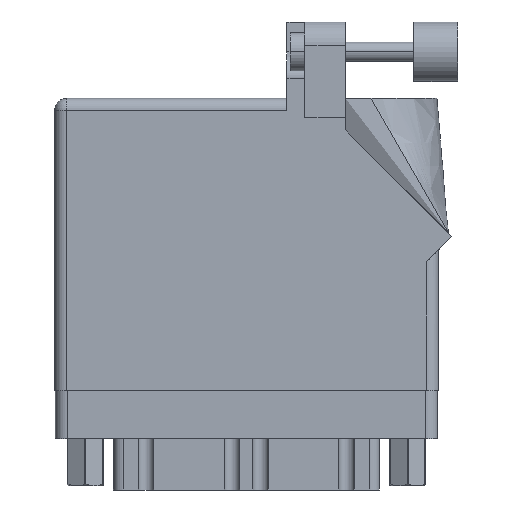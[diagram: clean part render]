
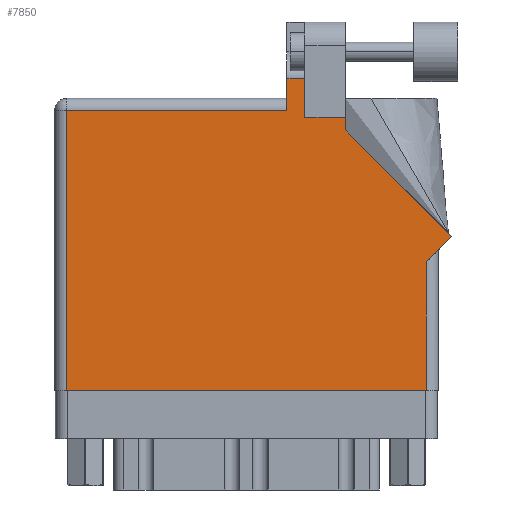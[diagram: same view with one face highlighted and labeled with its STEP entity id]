
A CAD part, front view. The second image highlights one B-rep face of the part: STEP entity #7850.
In plain terms, the highlighted face is planar.
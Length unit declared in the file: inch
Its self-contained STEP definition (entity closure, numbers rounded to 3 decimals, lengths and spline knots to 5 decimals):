
#1096 = CARTESIAN_POINT ( 'NONE',  ( 2.08071, 0.80771, 0. ) ) ;
#1359 = CARTESIAN_POINT ( 'NONE',  ( 1.64177, 1.6315, 0. ) ) ;
#1380 = DIRECTION ( 'NONE',  ( -0.707, 0.707, 0. ) ) ;
#2494 = ORIENTED_EDGE ( 'NONE', *, *, #47624, .T. ) ;
#3216 = ORIENTED_EDGE ( 'NONE', *, *, #21384, .T. ) ;
#3385 = CARTESIAN_POINT ( 'NONE',  ( 1.948, 0.675, 0. ) ) ;
#4133 = EDGE_CURVE ( 'NONE', #13836, #4342, #5826, .T. ) ;
#4342 = VERTEX_POINT ( 'NONE', #3385 ) ;
#4451 = LINE ( 'NONE', #30096, #24862 ) ;
#4482 = DIRECTION ( 'NONE',  ( -1., 0., 0. ) ) ;
#5068 = DIRECTION ( 'NONE',  ( 0., 1., 0. ) ) ;
#5462 = CARTESIAN_POINT ( 'NONE',  ( 0.062, 1.468, 0. ) ) ;
#5643 = VECTOR ( 'NONE', #34940, 39.37008 ) ;
#5826 = LINE ( 'NONE', #31470, #34584 ) ;
#6479 = EDGE_CURVE ( 'NONE', #15220, #13836, #27230, .T. ) ;
#6945 = DIRECTION ( 'NONE',  ( 0., -1., 0. ) ) ;
#7033 = DIRECTION ( 'NONE',  ( 0., 1., 0. ) ) ;
#7850 = ADVANCED_FACE ( 'NONE', ( #42167 ), #42419, .F. ) ;
#9872 = VERTEX_POINT ( 'NONE', #5462 ) ;
#10407 = VECTOR ( 'NONE', #34933, 39.37008 ) ;
#11691 = EDGE_CURVE ( 'NONE', #4342, #17733, #41701, .T. ) ;
#11889 = CARTESIAN_POINT ( 'NONE',  ( 1.524, 1.36442, 0. ) ) ;
#12659 = ORIENTED_EDGE ( 'NONE', *, *, #37640, .T. ) ;
#12720 = CARTESIAN_POINT ( 'NONE',  ( 2.01, 0.737, 0. ) ) ;
#12877 = EDGE_CURVE ( 'NONE', #14871, #16845, #34713, .T. ) ;
#13010 = EDGE_CURVE ( 'NONE', #38426, #9872, #4451, .T. ) ;
#13297 = CARTESIAN_POINT ( 'NONE',  ( 1.311, 1.43, 0. ) ) ;
#13383 = CARTESIAN_POINT ( 'NONE',  ( 0.062, 0., 0. ) ) ;
#13777 = VECTOR ( 'NONE', #1380, 39.37008 ) ;
#13836 = VERTEX_POINT ( 'NONE', #24693 ) ;
#14056 = VERTEX_POINT ( 'NONE', #13297 ) ;
#14092 = CARTESIAN_POINT ( 'NONE',  ( 1.311, 1.43, 0. ) ) ;
#14220 = CARTESIAN_POINT ( 'NONE',  ( 1.217, 1.53, 0. ) ) ;
#14871 = VERTEX_POINT ( 'NONE', #16991 ) ;
#15030 = CARTESIAN_POINT ( 'NONE',  ( 1.217, 1.468, 0. ) ) ;
#15220 = VERTEX_POINT ( 'NONE', #29746 ) ;
#15443 = CARTESIAN_POINT ( 'NONE',  ( 2.08071, 0.80771, 0. ) ) ;
#15795 = CARTESIAN_POINT ( 'NONE',  ( 1.217, 1.6315, 0. ) ) ;
#15937 = ORIENTED_EDGE ( 'NONE', *, *, #11691, .T. ) ;
#16026 = EDGE_CURVE ( 'NONE', #16845, #38426, #27973, .T. ) ;
#16798 = VECTOR ( 'NONE', #24099, 39.37008 ) ;
#16845 = VERTEX_POINT ( 'NONE', #15795 ) ;
#16991 = CARTESIAN_POINT ( 'NONE',  ( 1.311, 1.6315, 0. ) ) ;
#17019 = ORIENTED_EDGE ( 'NONE', *, *, #6479, .T. ) ;
#17733 = VERTEX_POINT ( 'NONE', #1096 ) ;
#18754 = DIRECTION ( 'NONE',  ( -1., 0., 0. ) ) ;
#19469 = ORIENTED_EDGE ( 'NONE', *, *, #4133, .T. ) ;
#21384 = EDGE_CURVE ( 'NONE', #38442, #27335, #23693, .T. ) ;
#22266 = LINE ( 'NONE', #14092, #25045 ) ;
#23335 = DIRECTION ( 'NONE',  ( -1., 0., 0. ) ) ;
#23693 = LINE ( 'NONE', #11889, #28614 ) ;
#24099 = DIRECTION ( 'NONE',  ( 1., 0., 0. ) ) ;
#24693 = CARTESIAN_POINT ( 'NONE',  ( 1.948, 0., 0. ) ) ;
#24862 = VECTOR ( 'NONE', #18754, 39.37008 ) ;
#25045 = VECTOR ( 'NONE', #7033, 39.37008 ) ;
#26982 = DIRECTION ( 'NONE',  ( 0., 0., -1. ) ) ;
#27230 = LINE ( 'NONE', #27473, #16798 ) ;
#27335 = VERTEX_POINT ( 'NONE', #37423 ) ;
#27473 = CARTESIAN_POINT ( 'NONE',  ( 0., 0., 0. ) ) ;
#27496 = ORIENTED_EDGE ( 'NONE', *, *, #16026, .T. ) ;
#27973 = LINE ( 'NONE', #14220, #28317 ) ;
#28317 = VECTOR ( 'NONE', #6945, 39.37008 ) ;
#28557 = DIRECTION ( 'NONE',  ( 0., 1., 0. ) ) ;
#28614 = VECTOR ( 'NONE', #5068, 39.37008 ) ;
#29233 = DIRECTION ( 'NONE',  ( 0., -1., 0. ) ) ;
#29746 = CARTESIAN_POINT ( 'NONE',  ( 0.062, 0., 0. ) ) ;
#29874 = LINE ( 'NONE', #33737, #35937 ) ;
#30096 = CARTESIAN_POINT ( 'NONE',  ( 0., 1.468, 0. ) ) ;
#30912 = EDGE_LOOP ( 'NONE', ( #37670, #34709, #27496, #45629, #12659, #17019, #19469, #15937, #2494, #3216, #44753 ) ) ;
#31470 = CARTESIAN_POINT ( 'NONE',  ( 1.948, 0.737, 0. ) ) ;
#33737 = CARTESIAN_POINT ( 'NONE',  ( 1.524, 1.43, 0. ) ) ;
#34584 = VECTOR ( 'NONE', #28557, 39.37008 ) ;
#34709 = ORIENTED_EDGE ( 'NONE', *, *, #12877, .T. ) ;
#34713 = LINE ( 'NONE', #1359, #5643 ) ;
#34726 = CARTESIAN_POINT ( 'NONE',  ( 1.524, 1.36442, 0. ) ) ;
#34933 = DIRECTION ( 'NONE',  ( 0.707, 0.707, 0. ) ) ;
#34940 = DIRECTION ( 'NONE',  ( -1., 0., 0. ) ) ;
#35590 = LINE ( 'NONE', #13383, #38371 ) ;
#35937 = VECTOR ( 'NONE', #4482, 39.37008 ) ;
#37423 = CARTESIAN_POINT ( 'NONE',  ( 1.524, 1.43, 0. ) ) ;
#37640 = EDGE_CURVE ( 'NONE', #9872, #15220, #35590, .T. ) ;
#37670 = ORIENTED_EDGE ( 'NONE', *, *, #43318, .T. ) ;
#38371 = VECTOR ( 'NONE', #29233, 39.37008 ) ;
#38426 = VERTEX_POINT ( 'NONE', #15030 ) ;
#38442 = VERTEX_POINT ( 'NONE', #34726 ) ;
#38545 = CARTESIAN_POINT ( 'NONE',  ( 0., 1.53, 0. ) ) ;
#41497 = LINE ( 'NONE', #15443, #13777 ) ;
#41701 = LINE ( 'NONE', #12720, #10407 ) ;
#42167 = FACE_OUTER_BOUND ( 'NONE', #30912, .T. ) ;
#42419 = PLANE ( 'NONE',  #43823 ) ;
#43318 = EDGE_CURVE ( 'NONE', #14056, #14871, #22266, .T. ) ;
#43823 = AXIS2_PLACEMENT_3D ( 'NONE', #38545, #26982, #23335 ) ;
#44386 = EDGE_CURVE ( 'NONE', #27335, #14056, #29874, .T. ) ;
#44753 = ORIENTED_EDGE ( 'NONE', *, *, #44386, .T. ) ;
#45629 = ORIENTED_EDGE ( 'NONE', *, *, #13010, .T. ) ;
#47624 = EDGE_CURVE ( 'NONE', #17733, #38442, #41497, .T. ) ;
